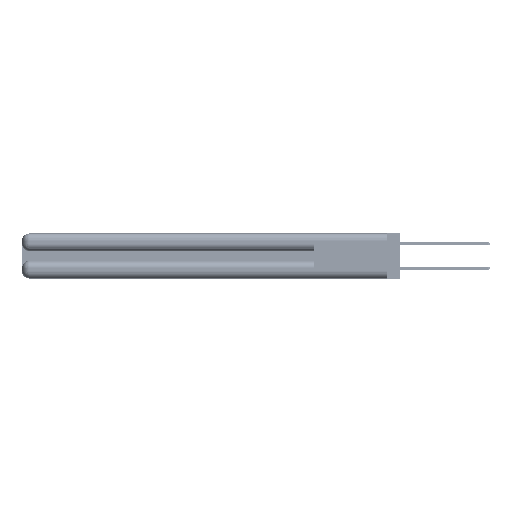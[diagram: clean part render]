
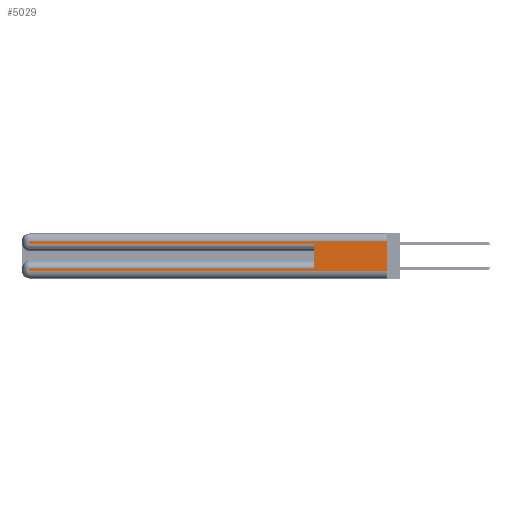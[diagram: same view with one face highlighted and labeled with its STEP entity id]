
A CAD part, left-side view. The second image highlights one B-rep face of the part: STEP entity #5029.
In plain terms, the highlighted planar face has unit normal (-1, 0, 0).
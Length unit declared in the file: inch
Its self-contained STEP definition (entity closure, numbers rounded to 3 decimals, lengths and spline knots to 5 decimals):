
#1285 = CARTESIAN_POINT ( 'NONE',  ( 0., 2.94, 0.37 ) ) ;
#1437 = VERTEX_POINT ( 'NONE', #36894 ) ;
#1704 = CARTESIAN_POINT ( 'NONE',  ( 0., 0., 0.37 ) ) ;
#2211 = VERTEX_POINT ( 'NONE', #46566 ) ;
#2488 = CARTESIAN_POINT ( 'NONE',  ( 0., 2.94, 0.285 ) ) ;
#4361 = ORIENTED_EDGE ( 'NONE', *, *, #30240, .T. ) ;
#4598 = CARTESIAN_POINT ( 'NONE',  ( 0., 0.6, 0.145 ) ) ;
#5029 = ADVANCED_FACE ( 'NONE', ( #40234 ), #27017, .F. ) ;
#5343 = DIRECTION ( 'NONE',  ( 0., -1., 0. ) ) ;
#5801 = EDGE_CURVE ( 'NONE', #26423, #23675, #49050, .T. ) ;
#6460 = CARTESIAN_POINT ( 'NONE',  ( 0., 0.6, 0.285 ) ) ;
#6908 = ORIENTED_EDGE ( 'NONE', *, *, #5801, .T. ) ;
#8689 = DIRECTION ( 'NONE',  ( 0., 0., 1. ) ) ;
#10562 = AXIS2_PLACEMENT_3D ( 'NONE', #48677, #44780, #40679 ) ;
#11450 = ORIENTED_EDGE ( 'NONE', *, *, #37753, .F. ) ;
#14356 = EDGE_LOOP ( 'NONE', ( #39279, #6908, #20856, #28237, #11450, #34665, #26306, #4361 ) ) ;
#18171 = EDGE_CURVE ( 'NONE', #28222, #2211, #44801, .T. ) ;
#19470 = VECTOR ( 'NONE', #41770, 39.37008 ) ;
#19843 = CARTESIAN_POINT ( 'NONE',  ( 0., 0., 0.085 ) ) ;
#20162 = DIRECTION ( 'NONE',  ( 0., 1., 0. ) ) ;
#20530 = DIRECTION ( 'NONE',  ( 0., 1., 0. ) ) ;
#20856 = ORIENTED_EDGE ( 'NONE', *, *, #37406, .T. ) ;
#21005 = EDGE_CURVE ( 'NONE', #26423, #37402, #22211, .T. ) ;
#22133 = DIRECTION ( 'NONE',  ( 0., 0., -1. ) ) ;
#22211 = LINE ( 'NONE', #1704, #42009 ) ;
#23675 = VERTEX_POINT ( 'NONE', #38357 ) ;
#24801 = VECTOR ( 'NONE', #8689, 39.37008 ) ;
#25711 = CARTESIAN_POINT ( 'NONE',  ( 0., 2.94, 0.37 ) ) ;
#26144 = LINE ( 'NONE', #4598, #24801 ) ;
#26306 = ORIENTED_EDGE ( 'NONE', *, *, #44305, .T. ) ;
#26423 = VERTEX_POINT ( 'NONE', #47998 ) ;
#27017 = PLANE ( 'NONE',  #10562 ) ;
#27078 = LINE ( 'NONE', #37660, #19470 ) ;
#28110 = LINE ( 'NONE', #25711, #44679 ) ;
#28222 = VERTEX_POINT ( 'NONE', #52297 ) ;
#28237 = ORIENTED_EDGE ( 'NONE', *, *, #34144, .T. ) ;
#29306 = CARTESIAN_POINT ( 'NONE',  ( 0., 0., 0.285 ) ) ;
#30240 = EDGE_CURVE ( 'NONE', #1437, #37402, #27078, .T. ) ;
#31425 = VECTOR ( 'NONE', #20530, 39.37008 ) ;
#32579 = CARTESIAN_POINT ( 'NONE',  ( 0., 0., 0.31 ) ) ;
#33573 = DIRECTION ( 'NONE',  ( 0., 0., -1. ) ) ;
#33732 = LINE ( 'NONE', #1285, #49666 ) ;
#34144 = EDGE_CURVE ( 'NONE', #50518, #43206, #52401, .T. ) ;
#34192 = DIRECTION ( 'NONE',  ( 0., 0., -1. ) ) ;
#34665 = ORIENTED_EDGE ( 'NONE', *, *, #18171, .T. ) ;
#36894 = CARTESIAN_POINT ( 'NONE',  ( 0., 2.94, 0.06 ) ) ;
#37402 = VERTEX_POINT ( 'NONE', #41253 ) ;
#37406 = EDGE_CURVE ( 'NONE', #23675, #50518, #33732, .T. ) ;
#37660 = CARTESIAN_POINT ( 'NONE',  ( 0., 0., 0.06 ) ) ;
#37753 = EDGE_CURVE ( 'NONE', #28222, #43206, #26144, .T. ) ;
#38357 = CARTESIAN_POINT ( 'NONE',  ( 0., 2.94, 0.31 ) ) ;
#39279 = ORIENTED_EDGE ( 'NONE', *, *, #21005, .F. ) ;
#40234 = FACE_OUTER_BOUND ( 'NONE', #14356, .T. ) ;
#40679 = DIRECTION ( 'NONE',  ( 0., 0., -1. ) ) ;
#41253 = CARTESIAN_POINT ( 'NONE',  ( 0., 0., 0.06 ) ) ;
#41579 = VECTOR ( 'NONE', #5343, 39.37008 ) ;
#41770 = DIRECTION ( 'NONE',  ( 0., -1., 0. ) ) ;
#42009 = VECTOR ( 'NONE', #34192, 39.37008 ) ;
#43206 = VERTEX_POINT ( 'NONE', #6460 ) ;
#44305 = EDGE_CURVE ( 'NONE', #2211, #1437, #28110, .T. ) ;
#44679 = VECTOR ( 'NONE', #22133, 39.37008 ) ;
#44780 = DIRECTION ( 'NONE',  ( 1., 0., 0. ) ) ;
#44801 = LINE ( 'NONE', #19843, #31425 ) ;
#46566 = CARTESIAN_POINT ( 'NONE',  ( 0., 2.94, 0.085 ) ) ;
#47792 = VECTOR ( 'NONE', #20162, 39.37008 ) ;
#47998 = CARTESIAN_POINT ( 'NONE',  ( 0., 0., 0.31 ) ) ;
#48677 = CARTESIAN_POINT ( 'NONE',  ( 0., 0., 0.37 ) ) ;
#49050 = LINE ( 'NONE', #32579, #47792 ) ;
#49666 = VECTOR ( 'NONE', #33573, 39.37008 ) ;
#50518 = VERTEX_POINT ( 'NONE', #2488 ) ;
#52297 = CARTESIAN_POINT ( 'NONE',  ( 0., 0.6, 0.085 ) ) ;
#52401 = LINE ( 'NONE', #29306, #41579 ) ;
